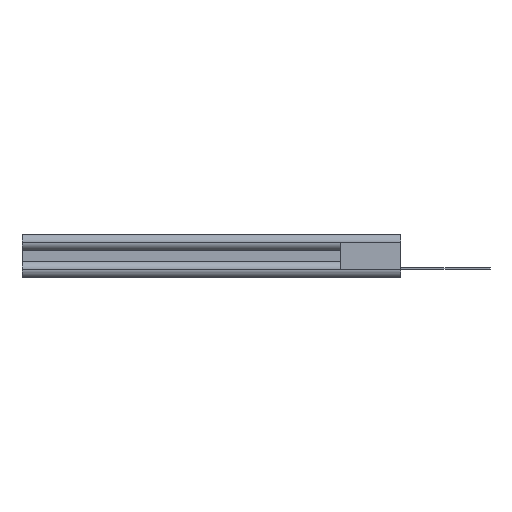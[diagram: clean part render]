
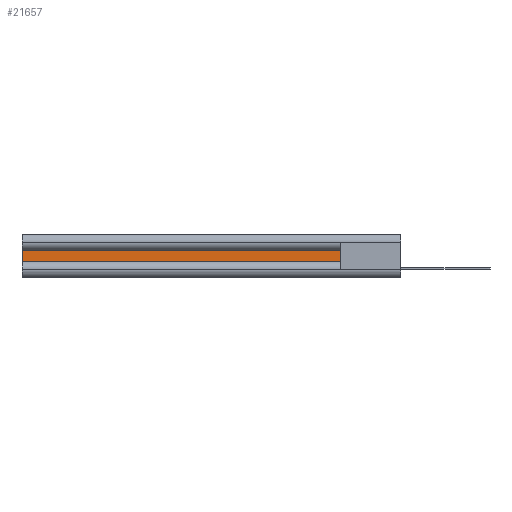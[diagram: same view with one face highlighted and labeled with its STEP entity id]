
A CAD part, left-side view. The second image highlights one B-rep face of the part: STEP entity #21657.
In plain terms, the highlighted planar face has unit normal (-1, 0, 0).
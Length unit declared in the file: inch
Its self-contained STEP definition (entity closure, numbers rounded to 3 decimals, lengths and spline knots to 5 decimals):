
#1357 = ORIENTED_EDGE ( 'NONE', *, *, #6391, .F. ) ;
#1514 = LINE ( 'NONE', #7971, #5609 ) ;
#1522 = LINE ( 'NONE', #4502, #5621 ) ;
#2425 = VERTEX_POINT ( 'NONE', #10992 ) ;
#3066 = LINE ( 'NONE', #12458, #7158 ) ;
#3814 = DIRECTION ( 'NONE',  ( 0., 0., -1. ) ) ;
#4502 = CARTESIAN_POINT ( 'NONE',  ( 0.044, 0.473, -0.0465 ) ) ;
#5138 = VERTEX_POINT ( 'NONE', #12140 ) ;
#5480 = CARTESIAN_POINT ( 'NONE',  ( 0.044, 0.473, -0.0465 ) ) ;
#5609 = VECTOR ( 'NONE', #14804, 39.37008 ) ;
#5621 = VECTOR ( 'NONE', #18132, 39.37008 ) ;
#6363 = PLANE ( 'NONE',  #10729 ) ;
#6391 = EDGE_CURVE ( 'NONE', #11170, #15329, #17448, .T. ) ;
#7158 = VECTOR ( 'NONE', #3814, 39.37008 ) ;
#7903 = VECTOR ( 'NONE', #17460, 39.37008 ) ;
#7971 = CARTESIAN_POINT ( 'NONE',  ( 0.044, 0.37012, 0.0465 ) ) ;
#8105 = CARTESIAN_POINT ( 'NONE',  ( 0.044, 0.37012, -0.0465 ) ) ;
#9226 = EDGE_CURVE ( 'NONE', #5138, #11170, #1522, .T. ) ;
#9825 = DIRECTION ( 'NONE',  ( 1., 0., 0. ) ) ;
#10194 = ORIENTED_EDGE ( 'NONE', *, *, #19187, .T. ) ;
#10525 = CARTESIAN_POINT ( 'NONE',  ( 0.044, 3., -0.0465 ) ) ;
#10729 = AXIS2_PLACEMENT_3D ( 'NONE', #8105, #9825, #21670 ) ;
#10992 = CARTESIAN_POINT ( 'NONE',  ( 0.044, 3., 0.0465 ) ) ;
#11170 = VERTEX_POINT ( 'NONE', #5480 ) ;
#11204 = EDGE_CURVE ( 'NONE', #2425, #15329, #3066, .T. ) ;
#11609 = EDGE_LOOP ( 'NONE', ( #10194, #13991, #1357, #17542 ) ) ;
#12140 = CARTESIAN_POINT ( 'NONE',  ( 0.044, 0.473, 0.0465 ) ) ;
#12458 = CARTESIAN_POINT ( 'NONE',  ( 0.044, 3., -0.0465 ) ) ;
#13991 = ORIENTED_EDGE ( 'NONE', *, *, #11204, .T. ) ;
#14334 = FACE_OUTER_BOUND ( 'NONE', #11609, .T. ) ;
#14804 = DIRECTION ( 'NONE',  ( 0., 1., 0. ) ) ;
#15329 = VERTEX_POINT ( 'NONE', #10525 ) ;
#15767 = CARTESIAN_POINT ( 'NONE',  ( 0.044, 0.37012, -0.0465 ) ) ;
#17448 = LINE ( 'NONE', #15767, #7903 ) ;
#17460 = DIRECTION ( 'NONE',  ( 0., 1., 0. ) ) ;
#17542 = ORIENTED_EDGE ( 'NONE', *, *, #9226, .F. ) ;
#18132 = DIRECTION ( 'NONE',  ( 0., 0., -1. ) ) ;
#19187 = EDGE_CURVE ( 'NONE', #5138, #2425, #1514, .T. ) ;
#21657 = ADVANCED_FACE ( 'NONE', ( #14334 ), #6363, .F. ) ;
#21670 = DIRECTION ( 'NONE',  ( 0., 0., -1. ) ) ;
